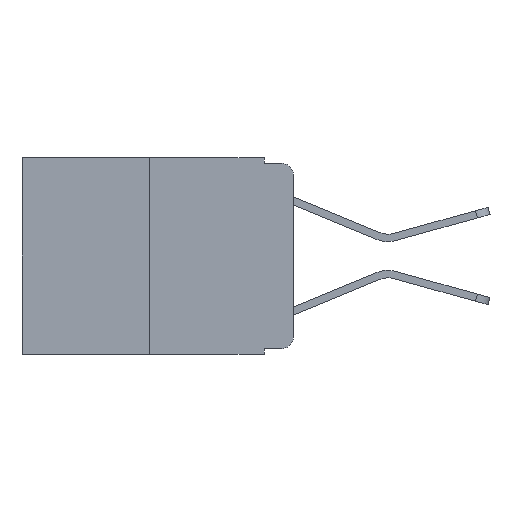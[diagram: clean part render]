
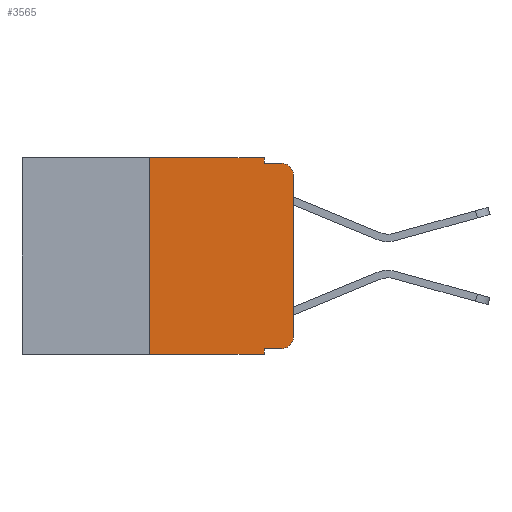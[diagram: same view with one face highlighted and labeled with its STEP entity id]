
A CAD part, left-side view. The second image highlights one B-rep face of the part: STEP entity #3565.
In plain terms, the highlighted planar face has unit normal (-1, 0, 0).
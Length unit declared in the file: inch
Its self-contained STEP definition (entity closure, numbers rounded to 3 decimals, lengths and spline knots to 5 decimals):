
#563 = ORIENTED_EDGE ( 'NONE', *, *, #4367, .F. ) ;
#564 = CARTESIAN_POINT ( 'NONE',  ( 0., 0.051, -0.343 ) ) ;
#699 = EDGE_CURVE ( 'NONE', #5211, #2709, #11526, .T. ) ;
#847 = DIRECTION ( 'NONE',  ( 0., 0., -1. ) ) ;
#1009 = AXIS2_PLACEMENT_3D ( 'NONE', #11129, #4959, #8821 ) ;
#1305 = VECTOR ( 'NONE', #847, 39.37008 ) ;
#1337 = DIRECTION ( 'NONE',  ( 0., -1., 0. ) ) ;
#1681 = LINE ( 'NONE', #5593, #11573 ) ;
#1911 = AXIS2_PLACEMENT_3D ( 'NONE', #10991, #5560, #11854 ) ;
#1999 = ORIENTED_EDGE ( 'NONE', *, *, #9284, .T. ) ;
#2068 = EDGE_CURVE ( 'NONE', #2709, #10985, #2694, .T. ) ;
#2553 = DIRECTION ( 'NONE',  ( 0., 0., 1. ) ) ;
#2597 = CARTESIAN_POINT ( 'NONE',  ( 0., 0.02, -0.313 ) ) ;
#2650 = VERTEX_POINT ( 'NONE', #4833 ) ;
#2679 = CIRCLE ( 'NONE', #1911, 0.02 ) ;
#2694 = CIRCLE ( 'NONE', #9146, 0.02 ) ;
#2709 = VERTEX_POINT ( 'NONE', #6731 ) ;
#2803 = DIRECTION ( 'NONE',  ( 0., 0., 1. ) ) ;
#2943 = LINE ( 'NONE', #4280, #10147 ) ;
#2987 = CARTESIAN_POINT ( 'NONE',  ( 0., 0.051, -0.333 ) ) ;
#3565 = ADVANCED_FACE ( 'NONE', ( #10960 ), #4964, .F. ) ;
#3710 = VERTEX_POINT ( 'NONE', #11366 ) ;
#3764 = DIRECTION ( 'NONE',  ( 0., -1., 0. ) ) ;
#3818 = CARTESIAN_POINT ( 'NONE',  ( 0., 0.051, 0. ) ) ;
#3853 = LINE ( 'NONE', #9167, #6664 ) ;
#4002 = ORIENTED_EDGE ( 'NONE', *, *, #9885, .T. ) ;
#4235 = CARTESIAN_POINT ( 'NONE',  ( 0., 0.051, 0. ) ) ;
#4280 = CARTESIAN_POINT ( 'NONE',  ( 0., 0.473, -0.343 ) ) ;
#4315 = EDGE_CURVE ( 'NONE', #8408, #8444, #2943, .T. ) ;
#4367 = EDGE_CURVE ( 'NONE', #9024, #11388, #9564, .T. ) ;
#4451 = ORIENTED_EDGE ( 'NONE', *, *, #699, .T. ) ;
#4612 = CARTESIAN_POINT ( 'NONE',  ( 0., 0., -0.313 ) ) ;
#4753 = ORIENTED_EDGE ( 'NONE', *, *, #2068, .T. ) ;
#4833 = CARTESIAN_POINT ( 'NONE',  ( 0., 0.02, -0.01 ) ) ;
#4959 = DIRECTION ( 'NONE',  ( 1., 0., 0. ) ) ;
#4964 = PLANE ( 'NONE',  #1009 ) ;
#5211 = VERTEX_POINT ( 'NONE', #9338 ) ;
#5560 = DIRECTION ( 'NONE',  ( -1., 0., 0. ) ) ;
#5593 = CARTESIAN_POINT ( 'NONE',  ( 0., 0.051, 0. ) ) ;
#6345 = LINE ( 'NONE', #6602, #10602 ) ;
#6423 = DIRECTION ( 'NONE',  ( 0., 0., -1. ) ) ;
#6436 = DIRECTION ( 'NONE',  ( -1., 0., 0. ) ) ;
#6602 = CARTESIAN_POINT ( 'NONE',  ( 0., 0.25, 0. ) ) ;
#6664 = VECTOR ( 'NONE', #2553, 39.37008 ) ;
#6713 = CARTESIAN_POINT ( 'NONE',  ( 0., 0., -0.03 ) ) ;
#6731 = CARTESIAN_POINT ( 'NONE',  ( 0., 0.02, -0.333 ) ) ;
#6752 = LINE ( 'NONE', #3818, #1305 ) ;
#7111 = DIRECTION ( 'NONE',  ( 0., -1., 0. ) ) ;
#7537 = LINE ( 'NONE', #7552, #9649 ) ;
#7552 = CARTESIAN_POINT ( 'NONE',  ( 0., 0.051, -0.01 ) ) ;
#8408 = VERTEX_POINT ( 'NONE', #10895 ) ;
#8444 = VERTEX_POINT ( 'NONE', #564 ) ;
#8552 = EDGE_LOOP ( 'NONE', ( #4002, #1999, #11847, #10121, #563, #10646, #11197, #11456, #4451, #4753 ) ) ;
#8821 = DIRECTION ( 'NONE',  ( 0., 0., -1. ) ) ;
#9024 = VERTEX_POINT ( 'NONE', #9777 ) ;
#9146 = AXIS2_PLACEMENT_3D ( 'NONE', #2597, #6436, #6423 ) ;
#9167 = CARTESIAN_POINT ( 'NONE',  ( 0., 0., 0. ) ) ;
#9199 = VECTOR ( 'NONE', #7111, 39.37008 ) ;
#9284 = EDGE_CURVE ( 'NONE', #11133, #2650, #2679, .T. ) ;
#9338 = CARTESIAN_POINT ( 'NONE',  ( 0., 0.051, -0.333 ) ) ;
#9564 = LINE ( 'NONE', #9952, #11608 ) ;
#9649 = VECTOR ( 'NONE', #3764, 39.37008 ) ;
#9777 = CARTESIAN_POINT ( 'NONE',  ( 0., 0.25, 0. ) ) ;
#9885 = EDGE_CURVE ( 'NONE', #10985, #11133, #3853, .T. ) ;
#9952 = CARTESIAN_POINT ( 'NONE',  ( 0., 0.473, 0. ) ) ;
#10121 = ORIENTED_EDGE ( 'NONE', *, *, #10481, .F. ) ;
#10147 = VECTOR ( 'NONE', #1337, 39.37008 ) ;
#10481 = EDGE_CURVE ( 'NONE', #11388, #3710, #1681, .T. ) ;
#10602 = VECTOR ( 'NONE', #2803, 39.37008 ) ;
#10646 = ORIENTED_EDGE ( 'NONE', *, *, #11622, .F. ) ;
#10828 = DIRECTION ( 'NONE',  ( 0., -1., 0. ) ) ;
#10895 = CARTESIAN_POINT ( 'NONE',  ( 0., 0.25, -0.343 ) ) ;
#10960 = FACE_OUTER_BOUND ( 'NONE', #8552, .T. ) ;
#10985 = VERTEX_POINT ( 'NONE', #4612 ) ;
#10991 = CARTESIAN_POINT ( 'NONE',  ( 0., 0.02, -0.03 ) ) ;
#11060 = EDGE_CURVE ( 'NONE', #3710, #2650, #7537, .T. ) ;
#11129 = CARTESIAN_POINT ( 'NONE',  ( 0., 0.473, 0. ) ) ;
#11133 = VERTEX_POINT ( 'NONE', #6713 ) ;
#11197 = ORIENTED_EDGE ( 'NONE', *, *, #4315, .T. ) ;
#11366 = CARTESIAN_POINT ( 'NONE',  ( 0., 0.051, -0.01 ) ) ;
#11388 = VERTEX_POINT ( 'NONE', #4235 ) ;
#11456 = ORIENTED_EDGE ( 'NONE', *, *, #12192, .F. ) ;
#11526 = LINE ( 'NONE', #2987, #9199 ) ;
#11573 = VECTOR ( 'NONE', #11899, 39.37008 ) ;
#11608 = VECTOR ( 'NONE', #10828, 39.37008 ) ;
#11622 = EDGE_CURVE ( 'NONE', #8408, #9024, #6345, .T. ) ;
#11847 = ORIENTED_EDGE ( 'NONE', *, *, #11060, .F. ) ;
#11854 = DIRECTION ( 'NONE',  ( 0., 0., -1. ) ) ;
#11899 = DIRECTION ( 'NONE',  ( 0., 0., -1. ) ) ;
#12192 = EDGE_CURVE ( 'NONE', #5211, #8444, #6752, .T. ) ;
